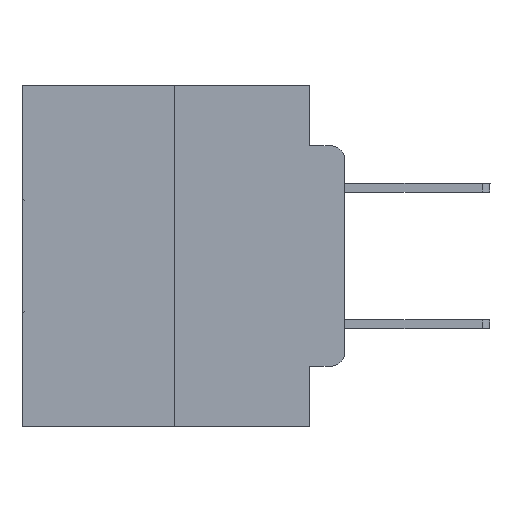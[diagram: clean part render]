
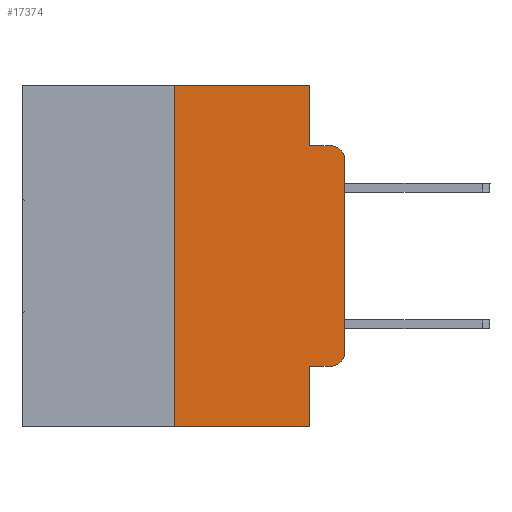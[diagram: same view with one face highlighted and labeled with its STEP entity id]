
A CAD part, left-side view. The second image highlights one B-rep face of the part: STEP entity #17374.
In plain terms, the highlighted planar face has unit normal (-1, 0, 0).
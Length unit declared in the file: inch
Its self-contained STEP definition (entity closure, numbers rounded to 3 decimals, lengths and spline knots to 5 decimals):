
#703 = VECTOR ( 'NONE', #3744, 39.37008 ) ;
#834 = CARTESIAN_POINT ( 'NONE',  ( 0., 0.473, 0. ) ) ;
#1063 = VERTEX_POINT ( 'NONE', #21559 ) ;
#1477 = CARTESIAN_POINT ( 'NONE',  ( 0., 0.25, 0. ) ) ;
#2470 = EDGE_CURVE ( 'NONE', #25185, #25932, #3729, .T. ) ;
#3074 = EDGE_CURVE ( 'NONE', #21211, #20608, #5383, .T. ) ;
#3474 = CARTESIAN_POINT ( 'NONE',  ( 0., 0., 0. ) ) ;
#3716 = ORIENTED_EDGE ( 'NONE', *, *, #26326, .T. ) ;
#3729 = LINE ( 'NONE', #13258, #5878 ) ;
#3744 = DIRECTION ( 'NONE',  ( 0., -1., 0. ) ) ;
#4309 = ORIENTED_EDGE ( 'NONE', *, *, #9838, .F. ) ;
#4355 = DIRECTION ( 'NONE',  ( 0., 0., -1. ) ) ;
#4889 = AXIS2_PLACEMENT_3D ( 'NONE', #26486, #9462, #23841 ) ;
#5078 = CARTESIAN_POINT ( 'NONE',  ( 0., 0.051, -0.5 ) ) ;
#5383 = CIRCLE ( 'NONE', #4889, 0.02 ) ;
#5755 = DIRECTION ( 'NONE',  ( 0., -1., 0. ) ) ;
#5878 = VECTOR ( 'NONE', #5755, 39.37008 ) ;
#6623 = DIRECTION ( 'NONE',  ( 0., -1., 0. ) ) ;
#7275 = EDGE_CURVE ( 'NONE', #10801, #9285, #27264, .T. ) ;
#7731 = EDGE_CURVE ( 'NONE', #25185, #12823, #12998, .T. ) ;
#8025 = DIRECTION ( 'NONE',  ( 1., 0., 0. ) ) ;
#8513 = CARTESIAN_POINT ( 'NONE',  ( 0., 0.051, 0. ) ) ;
#8613 = ORIENTED_EDGE ( 'NONE', *, *, #7731, .F. ) ;
#9281 = CIRCLE ( 'NONE', #17270, 0.02 ) ;
#9285 = VERTEX_POINT ( 'NONE', #24357 ) ;
#9462 = DIRECTION ( 'NONE',  ( -1., 0., 0. ) ) ;
#9733 = VECTOR ( 'NONE', #22832, 39.37008 ) ;
#9838 = EDGE_CURVE ( 'NONE', #29640, #25932, #15400, .T. ) ;
#10652 = DIRECTION ( 'NONE',  ( 0., 0., 1. ) ) ;
#10792 = LINE ( 'NONE', #13128, #9733 ) ;
#10801 = VERTEX_POINT ( 'NONE', #15792 ) ;
#12063 = ORIENTED_EDGE ( 'NONE', *, *, #20821, .T. ) ;
#12823 = VERTEX_POINT ( 'NONE', #1477 ) ;
#12998 = LINE ( 'NONE', #22536, #26022 ) ;
#13123 = VECTOR ( 'NONE', #18059, 39.37008 ) ;
#13128 = CARTESIAN_POINT ( 'NONE',  ( 0., 0.051, 0. ) ) ;
#13258 = CARTESIAN_POINT ( 'NONE',  ( 0., 0.473, -0.5 ) ) ;
#13323 = ORIENTED_EDGE ( 'NONE', *, *, #7275, .F. ) ;
#13543 = VERTEX_POINT ( 'NONE', #15031 ) ;
#14829 = CARTESIAN_POINT ( 'NONE',  ( 0., 0.02, -0.4115 ) ) ;
#15031 = CARTESIAN_POINT ( 'NONE',  ( 0., 0., -0.1085 ) ) ;
#15400 = LINE ( 'NONE', #8513, #13123 ) ;
#15717 = ORIENTED_EDGE ( 'NONE', *, *, #2470, .T. ) ;
#15792 = CARTESIAN_POINT ( 'NONE',  ( 0., 0.051, -0.0885 ) ) ;
#16229 = DIRECTION ( 'NONE',  ( -1., 0., 0. ) ) ;
#16312 = CARTESIAN_POINT ( 'NONE',  ( 0., 0.25, -0.5 ) ) ;
#17117 = EDGE_CURVE ( 'NONE', #12823, #1063, #20010, .T. ) ;
#17270 = AXIS2_PLACEMENT_3D ( 'NONE', #27502, #16229, #4355 ) ;
#17374 = ADVANCED_FACE ( 'NONE', ( #21941 ), #29130, .F. ) ;
#17568 = DIRECTION ( 'NONE',  ( 0., 0., -1. ) ) ;
#18047 = CARTESIAN_POINT ( 'NONE',  ( 0., 0.051, -0.0885 ) ) ;
#18059 = DIRECTION ( 'NONE',  ( 0., 0., -1. ) ) ;
#18515 = CARTESIAN_POINT ( 'NONE',  ( 0., 0.051, -0.4115 ) ) ;
#19522 = VECTOR ( 'NONE', #24757, 39.37008 ) ;
#19894 = LINE ( 'NONE', #3474, #22244 ) ;
#20010 = LINE ( 'NONE', #27351, #703 ) ;
#20197 = DIRECTION ( 'NONE',  ( 0., 0., 1. ) ) ;
#20233 = EDGE_CURVE ( 'NONE', #20608, #13543, #19894, .T. ) ;
#20514 = CARTESIAN_POINT ( 'NONE',  ( 0., 0.051, -0.4115 ) ) ;
#20608 = VERTEX_POINT ( 'NONE', #29215 ) ;
#20821 = EDGE_CURVE ( 'NONE', #13543, #9285, #9281, .T. ) ;
#21211 = VERTEX_POINT ( 'NONE', #14829 ) ;
#21559 = CARTESIAN_POINT ( 'NONE',  ( 0., 0.051, 0. ) ) ;
#21941 = FACE_OUTER_BOUND ( 'NONE', #28563, .T. ) ;
#22244 = VECTOR ( 'NONE', #20197, 39.37008 ) ;
#22536 = CARTESIAN_POINT ( 'NONE',  ( 0., 0.25, 0. ) ) ;
#22832 = DIRECTION ( 'NONE',  ( 0., 0., -1. ) ) ;
#23060 = ORIENTED_EDGE ( 'NONE', *, *, #28263, .F. ) ;
#23517 = ORIENTED_EDGE ( 'NONE', *, *, #20233, .T. ) ;
#23841 = DIRECTION ( 'NONE',  ( 0., 0., -1. ) ) ;
#24357 = CARTESIAN_POINT ( 'NONE',  ( 0., 0.02, -0.0885 ) ) ;
#24445 = ORIENTED_EDGE ( 'NONE', *, *, #17117, .F. ) ;
#24612 = VECTOR ( 'NONE', #6623, 39.37008 ) ;
#24757 = DIRECTION ( 'NONE',  ( 0., -1., 0. ) ) ;
#25165 = AXIS2_PLACEMENT_3D ( 'NONE', #834, #8025, #17568 ) ;
#25185 = VERTEX_POINT ( 'NONE', #16312 ) ;
#25932 = VERTEX_POINT ( 'NONE', #5078 ) ;
#26022 = VECTOR ( 'NONE', #10652, 39.37008 ) ;
#26326 = EDGE_CURVE ( 'NONE', #29640, #21211, #30218, .T. ) ;
#26486 = CARTESIAN_POINT ( 'NONE',  ( 0., 0.02, -0.3915 ) ) ;
#27264 = LINE ( 'NONE', #18047, #19522 ) ;
#27351 = CARTESIAN_POINT ( 'NONE',  ( 0., 0.473, 0. ) ) ;
#27502 = CARTESIAN_POINT ( 'NONE',  ( 0., 0.02, -0.1085 ) ) ;
#28263 = EDGE_CURVE ( 'NONE', #1063, #10801, #10792, .T. ) ;
#28563 = EDGE_LOOP ( 'NONE', ( #23517, #12063, #13323, #23060, #24445, #8613, #15717, #4309, #3716, #30481 ) ) ;
#29130 = PLANE ( 'NONE',  #25165 ) ;
#29215 = CARTESIAN_POINT ( 'NONE',  ( 0., 0., -0.3915 ) ) ;
#29640 = VERTEX_POINT ( 'NONE', #20514 ) ;
#30218 = LINE ( 'NONE', #18515, #24612 ) ;
#30481 = ORIENTED_EDGE ( 'NONE', *, *, #3074, .T. ) ;
